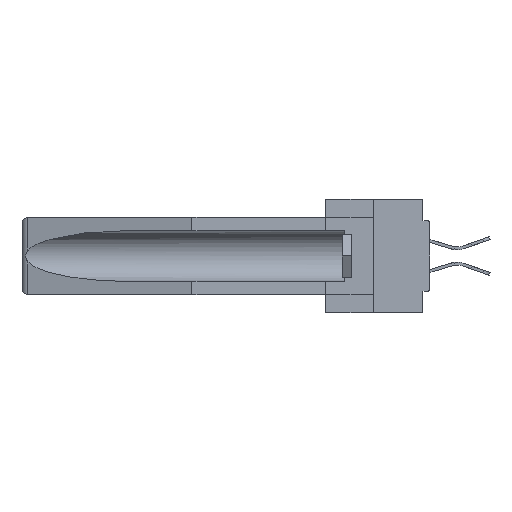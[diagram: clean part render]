
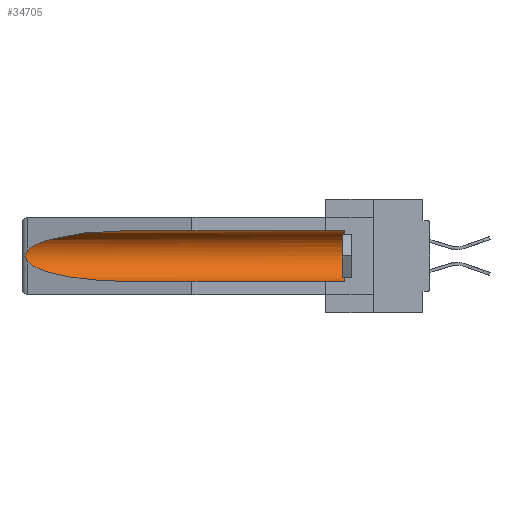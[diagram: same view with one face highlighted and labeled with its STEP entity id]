
A CAD part, left-side view. The second image highlights one B-rep face of the part: STEP entity #34705.
In plain terms, the highlighted cylindrical face has radius 2.857 mm (diameter 5.715 mm), a partial arc.
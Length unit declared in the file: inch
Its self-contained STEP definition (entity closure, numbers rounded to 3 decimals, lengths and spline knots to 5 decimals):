
#3465 = DIRECTION ( 'NONE',  ( 0., 1., 0. ) ) ;
#3754 = CARTESIAN_POINT ( 'NONE',  ( 0.26537, 1.52718, -0.14972 ) ) ;
#6210 = CARTESIAN_POINT ( 'NONE',  ( 0.26537, 1.52718, -0.19328 ) ) ;
#6377 = ORIENTED_EDGE ( 'NONE', *, *, #25756, .F. ) ;
#7061 = CARTESIAN_POINT ( 'NONE',  ( 0.155, -0.30754, -0.1715 ) ) ;
#7368 = DIRECTION ( 'NONE',  ( 0., 0., 1. ) ) ;
#8482 = CARTESIAN_POINT ( 'NONE',  ( 0.155, -0.30754, -0.059 ) ) ;
#8525 = ORIENTED_EDGE ( 'NONE', *, *, #40124, .T. ) ;
#8871 = ORIENTED_EDGE ( 'NONE', *, *, #30328, .T. ) ;
#10302 = CARTESIAN_POINT ( 'NONE',  ( 0.155, 1.07973, -0.284 ) ) ;
#10831 = ORIENTED_EDGE ( 'NONE', *, *, #10843, .T. ) ;
#10843 = EDGE_CURVE ( 'NONE', #20765, #41705, #15218, .T. ) ;
#11181 = CARTESIAN_POINT ( 'NONE',  ( 0.155, 0.126, -0.284 ) ) ;
#12459 = CIRCLE ( 'NONE', #44352, 0.1125 ) ;
#12830 = CARTESIAN_POINT ( 'NONE',  ( 0.26654, 1.53092, -0.15636 ) ) ;
#13073 = CARTESIAN_POINT ( 'NONE',  ( 0.155, 0.126, -0.1715 ) ) ;
#13139 = CARTESIAN_POINT ( 'NONE',  ( 0.2673, 1.5327, -0.16383 ) ) ;
#13220 = DIRECTION ( 'NONE',  ( 0., -1., 0. ) ) ;
#14502 = VERTEX_POINT ( 'NONE', #24938 ) ;
#15218 =( BOUNDED_CURVE ( )  B_SPLINE_CURVE ( 3, ( #20755, #38517, #17542, #10302 ),
 .UNSPECIFIED., .F., .F. ) 
 B_SPLINE_CURVE_WITH_KNOTS ( ( 4, 4 ),
 ( 0.1948, 1.5708 ),
 .UNSPECIFIED. ) 
 CURVE ( )  GEOMETRIC_REPRESENTATION_ITEM ( )  RATIONAL_B_SPLINE_CURVE ( ( 1., 0.848, 0.848, 1. ) ) 
 REPRESENTATION_ITEM ( '' )  );
#15287 = CARTESIAN_POINT ( 'NONE',  ( 0.26537, 1.52718, -0.19328 ) ) ;
#16405 = CARTESIAN_POINT ( 'NONE',  ( 0.2675, 1.53308, -0.17534 ) ) ;
#17542 = CARTESIAN_POINT ( 'NONE',  ( 0.21114, 1.30732, -0.284 ) ) ;
#18583 = CARTESIAN_POINT ( 'NONE',  ( 0.155, -0.30754, -0.284 ) ) ;
#19705 = B_SPLINE_CURVE_WITH_KNOTS ( 'NONE', 3,
 ( #20059, #34562, #12830, #13139, #23490, #16405, #41074, #19906, #20216, #6210 ),
 .UNSPECIFIED., .F., .F.,
 ( 4, 2, 2, 2, 4 ),
 ( 0., 0.00029, 0.00058, 0.00087, 0.00117 ),
 .UNSPECIFIED. ) ;
#19906 = CARTESIAN_POINT ( 'NONE',  ( 0.26655, 1.53094, -0.18657 ) ) ;
#20059 = CARTESIAN_POINT ( 'NONE',  ( 0.26537, 1.52718, -0.14972 ) ) ;
#20216 = CARTESIAN_POINT ( 'NONE',  ( 0.26597, 1.5296, -0.19026 ) ) ;
#20495 = CARTESIAN_POINT ( 'NONE',  ( 0.26537, 1.52718, -0.14972 ) ) ;
#20755 = CARTESIAN_POINT ( 'NONE',  ( 0.26537, 1.52718, -0.19328 ) ) ;
#20765 = VERTEX_POINT ( 'NONE', #15287 ) ;
#21669 = LINE ( 'NONE', #18583, #30489 ) ;
#23160 = EDGE_CURVE ( 'NONE', #28312, #14502, #28432, .T. ) ;
#23490 = CARTESIAN_POINT ( 'NONE',  ( 0.2675, 1.53308, -0.16763 ) ) ;
#24565 = CARTESIAN_POINT ( 'NONE',  ( 0.155, 0.126, -0.059 ) ) ;
#24938 = CARTESIAN_POINT ( 'NONE',  ( 0.155, 1.07973, -0.059 ) ) ;
#25756 = EDGE_CURVE ( 'NONE', #42044, #41705, #21669, .T. ) ;
#26096 = EDGE_CURVE ( 'NONE', #40694, #20765, #19705, .T. ) ;
#26778 = DIRECTION ( 'NONE',  ( 0., 1., 0. ) ) ;
#26891 = CARTESIAN_POINT ( 'NONE',  ( 0.25451, 1.48313, -0.09465 ) ) ;
#27560 = ORIENTED_EDGE ( 'NONE', *, *, #26096, .T. ) ;
#28312 = VERTEX_POINT ( 'NONE', #24565 ) ;
#28432 = LINE ( 'NONE', #8482, #35035 ) ;
#29339 = DIRECTION ( 'NONE',  ( 0., 1., 0. ) ) ;
#30328 = EDGE_CURVE ( 'NONE', #14502, #40694, #40396, .T. ) ;
#30344 = CYLINDRICAL_SURFACE ( 'NONE', #32663, 0.1125 ) ;
#30489 = VECTOR ( 'NONE', #29339, 39.37008 ) ;
#32568 = FACE_OUTER_BOUND ( 'NONE', #32673, .T. ) ;
#32663 = AXIS2_PLACEMENT_3D ( 'NONE', #7061, #3465, #7368 ) ;
#32673 = EDGE_LOOP ( 'NONE', ( #8871, #27560, #10831, #6377, #8525, #43604 ) ) ;
#33700 = DIRECTION ( 'NONE',  ( 0., 0., 1. ) ) ;
#34562 = CARTESIAN_POINT ( 'NONE',  ( 0.26597, 1.52961, -0.15275 ) ) ;
#34705 = ADVANCED_FACE ( 'NONE', ( #32568 ), #30344, .F. ) ;
#35035 = VECTOR ( 'NONE', #26778, 39.37008 ) ;
#38517 = CARTESIAN_POINT ( 'NONE',  ( 0.25451, 1.48313, -0.24835 ) ) ;
#40124 = EDGE_CURVE ( 'NONE', #42044, #28312, #12459, .T. ) ;
#40396 =( BOUNDED_CURVE ( )  B_SPLINE_CURVE ( 3, ( #40935, #44468, #26891, #3754 ),
 .UNSPECIFIED., .F., .F. ) 
 B_SPLINE_CURVE_WITH_KNOTS ( ( 4, 4 ),
 ( 4.71239, 6.08839 ),
 .UNSPECIFIED. ) 
 CURVE ( )  GEOMETRIC_REPRESENTATION_ITEM ( )  RATIONAL_B_SPLINE_CURVE ( ( 1., 0.848, 0.848, 1. ) ) 
 REPRESENTATION_ITEM ( '' )  );
#40694 = VERTEX_POINT ( 'NONE', #20495 ) ;
#40935 = CARTESIAN_POINT ( 'NONE',  ( 0.155, 1.07973, -0.059 ) ) ;
#41074 = CARTESIAN_POINT ( 'NONE',  ( 0.2673, 1.53269, -0.17917 ) ) ;
#41705 = VERTEX_POINT ( 'NONE', #43394 ) ;
#42044 = VERTEX_POINT ( 'NONE', #11181 ) ;
#43394 = CARTESIAN_POINT ( 'NONE',  ( 0.155, 1.07973, -0.284 ) ) ;
#43604 = ORIENTED_EDGE ( 'NONE', *, *, #23160, .T. ) ;
#44352 = AXIS2_PLACEMENT_3D ( 'NONE', #13073, #13220, #33700 ) ;
#44468 = CARTESIAN_POINT ( 'NONE',  ( 0.21114, 1.30732, -0.059 ) ) ;
